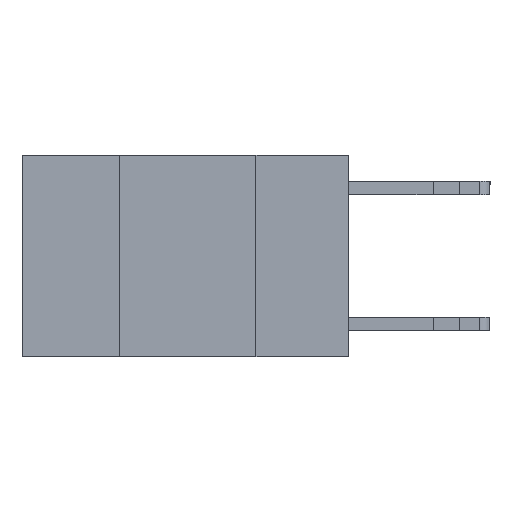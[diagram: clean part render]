
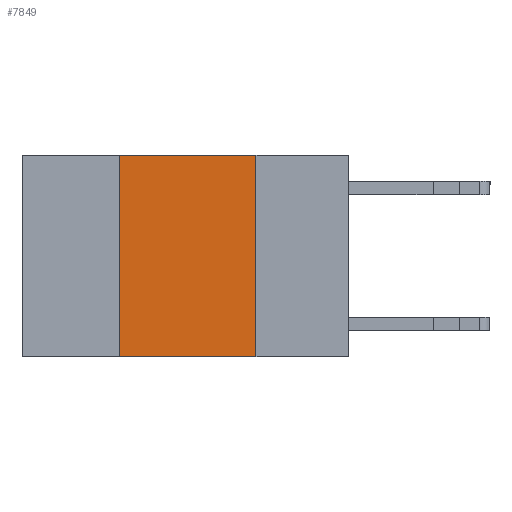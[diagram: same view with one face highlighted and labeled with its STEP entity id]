
A CAD part, left-side view. The second image highlights one B-rep face of the part: STEP entity #7849.
In plain terms, the highlighted planar face has unit normal (-1, 0, 0).
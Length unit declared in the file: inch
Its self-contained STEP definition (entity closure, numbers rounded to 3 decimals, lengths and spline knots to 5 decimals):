
#649 = VERTEX_POINT ( 'NONE', #15415 ) ;
#2009 = EDGE_CURVE ( 'NONE', #649, #3749, #16328, .T. ) ;
#2670 = CARTESIAN_POINT ( 'NONE',  ( 0., 0.42, -0.37 ) ) ;
#2835 = AXIS2_PLACEMENT_3D ( 'NONE', #8936, #3121, #16888 ) ;
#2852 = LINE ( 'NONE', #4568, #17494 ) ;
#3121 = DIRECTION ( 'NONE',  ( 1., 0., 0. ) ) ;
#3408 = DIRECTION ( 'NONE',  ( 0., 0., 1. ) ) ;
#3749 = VERTEX_POINT ( 'NONE', #12353 ) ;
#4004 = CARTESIAN_POINT ( 'NONE',  ( 0., 0.17, 0. ) ) ;
#4132 = ORIENTED_EDGE ( 'NONE', *, *, #7304, .F. ) ;
#4568 = CARTESIAN_POINT ( 'NONE',  ( 0., 0.6, -0.37 ) ) ;
#4707 = VERTEX_POINT ( 'NONE', #2670 ) ;
#5027 = LINE ( 'NONE', #5205, #12439 ) ;
#5205 = CARTESIAN_POINT ( 'NONE',  ( 0., 0.42, 0. ) ) ;
#5474 = ORIENTED_EDGE ( 'NONE', *, *, #2009, .F. ) ;
#5995 = VECTOR ( 'NONE', #12690, 39.37008 ) ;
#7077 = CARTESIAN_POINT ( 'NONE',  ( 0., 0.6, 0. ) ) ;
#7304 = EDGE_CURVE ( 'NONE', #12015, #649, #16647, .T. ) ;
#7316 = DIRECTION ( 'NONE',  ( 0., -1., 0. ) ) ;
#7494 = PLANE ( 'NONE',  #2835 ) ;
#7545 = ORIENTED_EDGE ( 'NONE', *, *, #10211, .F. ) ;
#7585 = CARTESIAN_POINT ( 'NONE',  ( 0., 0.42, 0. ) ) ;
#7849 = ADVANCED_FACE ( 'NONE', ( #10216 ), #7494, .F. ) ;
#8936 = CARTESIAN_POINT ( 'NONE',  ( 0., 0.6, 0. ) ) ;
#10211 = EDGE_CURVE ( 'NONE', #4707, #12015, #5027, .T. ) ;
#10216 = FACE_OUTER_BOUND ( 'NONE', #15646, .T. ) ;
#12015 = VERTEX_POINT ( 'NONE', #7585 ) ;
#12353 = CARTESIAN_POINT ( 'NONE',  ( 0., 0.17, -0.37 ) ) ;
#12439 = VECTOR ( 'NONE', #3408, 39.37008 ) ;
#12690 = DIRECTION ( 'NONE',  ( 0., -1., 0. ) ) ;
#14635 = ORIENTED_EDGE ( 'NONE', *, *, #16812, .T. ) ;
#15077 = DIRECTION ( 'NONE',  ( 0., 0., -1. ) ) ;
#15415 = CARTESIAN_POINT ( 'NONE',  ( 0., 0.17, 0. ) ) ;
#15510 = VECTOR ( 'NONE', #15077, 39.37008 ) ;
#15646 = EDGE_LOOP ( 'NONE', ( #5474, #4132, #7545, #14635 ) ) ;
#16328 = LINE ( 'NONE', #4004, #15510 ) ;
#16647 = LINE ( 'NONE', #7077, #5995 ) ;
#16812 = EDGE_CURVE ( 'NONE', #4707, #3749, #2852, .T. ) ;
#16888 = DIRECTION ( 'NONE',  ( 0., 0., -1. ) ) ;
#17494 = VECTOR ( 'NONE', #7316, 39.37008 ) ;
